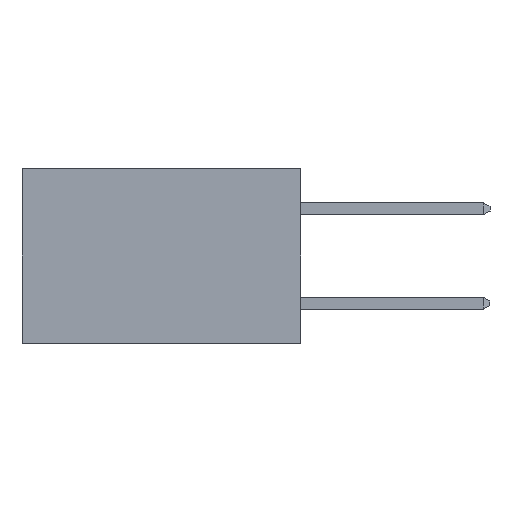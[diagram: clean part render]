
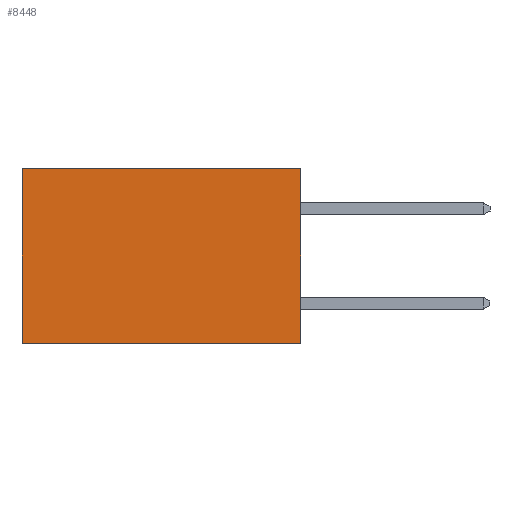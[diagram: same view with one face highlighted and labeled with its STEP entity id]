
A CAD part, left-side view. The second image highlights one B-rep face of the part: STEP entity #8448.
In plain terms, the highlighted planar face has unit normal (-1, 0, 0).
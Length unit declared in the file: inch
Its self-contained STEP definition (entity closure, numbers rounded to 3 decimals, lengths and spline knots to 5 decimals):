
#41 = CARTESIAN_POINT ( 'NONE',  ( 0.277, 0., -0.37 ) ) ;
#76 = CARTESIAN_POINT ( 'NONE',  ( 0.277, 0.59, -0.37 ) ) ;
#496 = CARTESIAN_POINT ( 'NONE',  ( 0.277, 0., -0.37 ) ) ;
#758 = ORIENTED_EDGE ( 'NONE', *, *, #1173, .T. ) ;
#831 = VECTOR ( 'NONE', #10019, 39.37008 ) ;
#857 = EDGE_CURVE ( 'NONE', #5126, #3763, #1293, .T. ) ;
#861 = ORIENTED_EDGE ( 'NONE', *, *, #7822, .F. ) ;
#884 = DIRECTION ( 'NONE',  ( 0., 0., -1. ) ) ;
#915 = ORIENTED_EDGE ( 'NONE', *, *, #857, .F. ) ;
#1053 = ORIENTED_EDGE ( 'NONE', *, *, #4618, .T. ) ;
#1173 = EDGE_CURVE ( 'NONE', #1988, #2756, #8557, .T. ) ;
#1293 = LINE ( 'NONE', #8997, #9631 ) ;
#1988 = VERTEX_POINT ( 'NONE', #9223 ) ;
#2460 = FACE_OUTER_BOUND ( 'NONE', #4930, .T. ) ;
#2756 = VERTEX_POINT ( 'NONE', #9262 ) ;
#3070 = VECTOR ( 'NONE', #7992, 39.37008 ) ;
#3763 = VERTEX_POINT ( 'NONE', #496 ) ;
#4618 = EDGE_CURVE ( 'NONE', #5126, #1988, #5149, .T. ) ;
#4930 = EDGE_LOOP ( 'NONE', ( #758, #861, #915, #1053 ) ) ;
#4945 = PLANE ( 'NONE',  #9305 ) ;
#5126 = VERTEX_POINT ( 'NONE', #6171 ) ;
#5149 = LINE ( 'NONE', #9364, #831 ) ;
#5209 = DIRECTION ( 'NONE',  ( 0., 0., -1. ) ) ;
#5730 = DIRECTION ( 'NONE',  ( 1., 0., 0. ) ) ;
#6171 = CARTESIAN_POINT ( 'NONE',  ( 0.277, 0., 0. ) ) ;
#6400 = DIRECTION ( 'NONE',  ( 0., 0., -1. ) ) ;
#7224 = CARTESIAN_POINT ( 'NONE',  ( 0.277, 0., -0.37 ) ) ;
#7822 = EDGE_CURVE ( 'NONE', #3763, #2756, #9285, .T. ) ;
#7992 = DIRECTION ( 'NONE',  ( 0., 1., 0. ) ) ;
#8314 = VECTOR ( 'NONE', #6400, 39.37008 ) ;
#8448 = ADVANCED_FACE ( 'NONE', ( #2460 ), #4945, .F. ) ;
#8557 = LINE ( 'NONE', #76, #8314 ) ;
#8997 = CARTESIAN_POINT ( 'NONE',  ( 0.277, 0., -0.37 ) ) ;
#9223 = CARTESIAN_POINT ( 'NONE',  ( 0.277, 0.59, 0. ) ) ;
#9262 = CARTESIAN_POINT ( 'NONE',  ( 0.277, 0.59, -0.37 ) ) ;
#9285 = LINE ( 'NONE', #7224, #3070 ) ;
#9305 = AXIS2_PLACEMENT_3D ( 'NONE', #41, #5730, #884 ) ;
#9364 = CARTESIAN_POINT ( 'NONE',  ( 0.277, 0., 0. ) ) ;
#9631 = VECTOR ( 'NONE', #5209, 39.37008 ) ;
#10019 = DIRECTION ( 'NONE',  ( 0., 1., 0. ) ) ;
